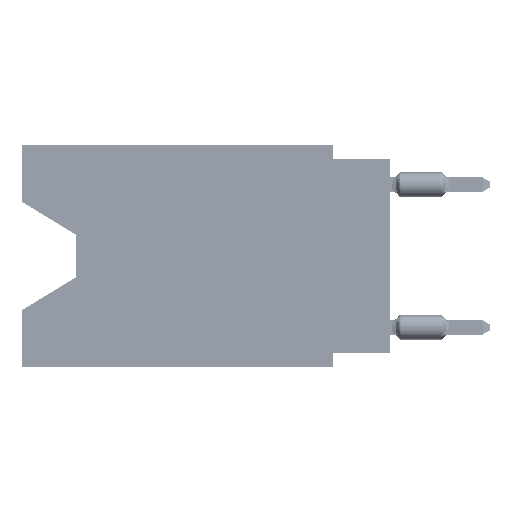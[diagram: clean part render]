
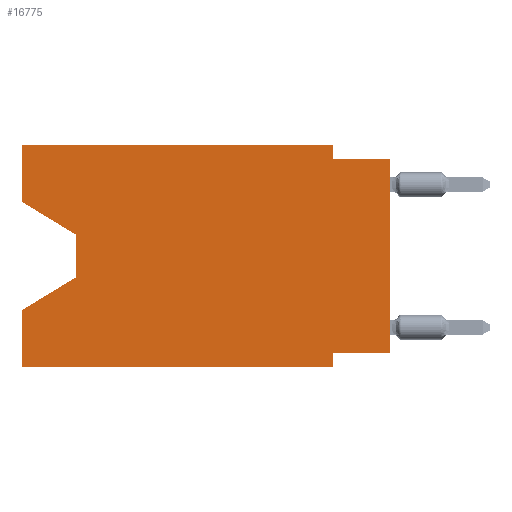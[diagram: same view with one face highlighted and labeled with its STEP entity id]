
A CAD part, left-side view. The second image highlights one B-rep face of the part: STEP entity #16775.
In plain terms, the highlighted planar face has unit normal (-1, 0, 0).
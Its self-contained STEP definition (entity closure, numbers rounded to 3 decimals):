
#1108 = CARTESIAN_POINT ( 'NONE',  ( 0., 16.383, -7.36 ) ) ;
#1515 = VECTOR ( 'NONE', #27946, 1000. ) ;
#1845 = EDGE_CURVE ( 'NONE', #78045, #65738, #79891, .T. ) ;
#3130 = CARTESIAN_POINT ( 'NONE',  ( 0., 16.383, 0. ) ) ;
#3333 = EDGE_CURVE ( 'NONE', #61982, #33048, #48291, .T. ) ;
#3709 = CARTESIAN_POINT ( 'NONE',  ( 0., 2.54, 0. ) ) ;
#4247 = LINE ( 'NONE', #18133, #17586 ) ;
#6754 = EDGE_CURVE ( 'NONE', #19609, #62767, #4247, .T. ) ;
#7972 = LINE ( 'NONE', #22274, #1515 ) ;
#8354 = DIRECTION ( 'NONE',  ( 0., 0., -1. ) ) ;
#8717 = LINE ( 'NONE', #36454, #43892 ) ;
#9831 = VECTOR ( 'NONE', #17596, 1000. ) ;
#12646 = CARTESIAN_POINT ( 'NONE',  ( 0., 16.383, 0. ) ) ;
#13495 = CARTESIAN_POINT ( 'NONE',  ( 0., 0., -0.635 ) ) ;
#13718 = CARTESIAN_POINT ( 'NONE',  ( 0., 13.97, -5.893 ) ) ;
#15014 = DIRECTION ( 'NONE',  ( 0., -1., 0. ) ) ;
#16775 = ADVANCED_FACE ( 'NONE', ( #78257 ), #64792, .F. ) ;
#17586 = VECTOR ( 'NONE', #44601, 1000. ) ;
#17596 = DIRECTION ( 'NONE',  ( 0., 0., -1. ) ) ;
#18133 = CARTESIAN_POINT ( 'NONE',  ( 0., 13.97, -4.013 ) ) ;
#18489 = VECTOR ( 'NONE', #82937, 1000. ) ;
#18749 = DIRECTION ( 'NONE',  ( 0., 0., -1. ) ) ;
#18790 = ORIENTED_EDGE ( 'NONE', *, *, #85277, .T. ) ;
#19493 = ORIENTED_EDGE ( 'NONE', *, *, #3333, .F. ) ;
#19609 = VERTEX_POINT ( 'NONE', #43507 ) ;
#20093 = CARTESIAN_POINT ( 'NONE',  ( 0., 2.54, -9.906 ) ) ;
#20587 = VECTOR ( 'NONE', #29185, 1000. ) ;
#20881 = ORIENTED_EDGE ( 'NONE', *, *, #49414, .F. ) ;
#21984 = EDGE_CURVE ( 'NONE', #61050, #45121, #60635, .T. ) ;
#22274 = CARTESIAN_POINT ( 'NONE',  ( 0., 0., -9.271 ) ) ;
#24250 = CARTESIAN_POINT ( 'NONE',  ( 0., 2.54, -9.271 ) ) ;
#24397 = LINE ( 'NONE', #49589, #58509 ) ;
#25466 = LINE ( 'NONE', #13718, #51421 ) ;
#25630 = ORIENTED_EDGE ( 'NONE', *, *, #6754, .T. ) ;
#26469 = CARTESIAN_POINT ( 'NONE',  ( 0., 2.54, 0. ) ) ;
#27946 = DIRECTION ( 'NONE',  ( 0., 1., 0. ) ) ;
#28156 = DIRECTION ( 'NONE',  ( 0., 0., 1. ) ) ;
#29185 = DIRECTION ( 'NONE',  ( 0., -1., 0. ) ) ;
#30332 = LINE ( 'NONE', #49467, #18489 ) ;
#33048 = VERTEX_POINT ( 'NONE', #20093 ) ;
#33711 = CARTESIAN_POINT ( 'NONE',  ( 0., 16.383, 0. ) ) ;
#33795 = CARTESIAN_POINT ( 'NONE',  ( 0., 16.383, 0. ) ) ;
#36454 = CARTESIAN_POINT ( 'NONE',  ( 0., 0., 0. ) ) ;
#36660 = LINE ( 'NONE', #48002, #85821 ) ;
#36768 = ORIENTED_EDGE ( 'NONE', *, *, #56775, .T. ) ;
#37767 = VERTEX_POINT ( 'NONE', #26469 ) ;
#38021 = VECTOR ( 'NONE', #28156, 1000. ) ;
#41029 = ORIENTED_EDGE ( 'NONE', *, *, #65079, .T. ) ;
#41229 = ORIENTED_EDGE ( 'NONE', *, *, #1845, .F. ) ;
#43507 = CARTESIAN_POINT ( 'NONE',  ( 0., 13.97, -4.013 ) ) ;
#43892 = VECTOR ( 'NONE', #61683, 1000. ) ;
#43999 = CARTESIAN_POINT ( 'NONE',  ( 0., 16.383, -9.906 ) ) ;
#44601 = DIRECTION ( 'NONE',  ( 0., 0., -1. ) ) ;
#45121 = VERTEX_POINT ( 'NONE', #1108 ) ;
#46500 = EDGE_CURVE ( 'NONE', #37767, #75358, #50590, .T. ) ;
#46737 = EDGE_CURVE ( 'NONE', #79454, #61982, #7972, .T. ) ;
#46905 = EDGE_CURVE ( 'NONE', #62767, #45121, #25466, .T. ) ;
#47860 = CARTESIAN_POINT ( 'NONE',  ( 0., 2.54, -9.906 ) ) ;
#48002 = CARTESIAN_POINT ( 'NONE',  ( 0., 16.383, -9.906 ) ) ;
#48291 = LINE ( 'NONE', #47860, #64580 ) ;
#48818 = CARTESIAN_POINT ( 'NONE',  ( 0., 0., -9.271 ) ) ;
#49414 = EDGE_CURVE ( 'NONE', #75358, #72971, #30332, .T. ) ;
#49467 = CARTESIAN_POINT ( 'NONE',  ( 0., 0., -0.635 ) ) ;
#49589 = CARTESIAN_POINT ( 'NONE',  ( 0., 16.383, -2.546 ) ) ;
#50590 = LINE ( 'NONE', #3709, #9831 ) ;
#50895 = DIRECTION ( 'NONE',  ( 0., -0.855, -0.519 ) ) ;
#51421 = VECTOR ( 'NONE', #79323, 1000. ) ;
#52121 = ORIENTED_EDGE ( 'NONE', *, *, #46737, .F. ) ;
#56775 = EDGE_CURVE ( 'NONE', #79454, #72971, #8717, .T. ) ;
#56961 = ORIENTED_EDGE ( 'NONE', *, *, #46500, .F. ) ;
#58368 = ORIENTED_EDGE ( 'NONE', *, *, #21984, .F. ) ;
#58509 = VECTOR ( 'NONE', #50895, 1000. ) ;
#59257 = EDGE_CURVE ( 'NONE', #65738, #37767, #69573, .T. ) ;
#59350 = DIRECTION ( 'NONE',  ( 0., 0., 1. ) ) ;
#59527 = AXIS2_PLACEMENT_3D ( 'NONE', #12646, #64355, #18749 ) ;
#60635 = LINE ( 'NONE', #33711, #68288 ) ;
#61050 = VERTEX_POINT ( 'NONE', #43999 ) ;
#61683 = DIRECTION ( 'NONE',  ( 0., 0., 1. ) ) ;
#61982 = VERTEX_POINT ( 'NONE', #24250 ) ;
#62767 = VERTEX_POINT ( 'NONE', #69658 ) ;
#64355 = DIRECTION ( 'NONE',  ( 1., 0., 0. ) ) ;
#64580 = VECTOR ( 'NONE', #8354, 1000. ) ;
#64792 = PLANE ( 'NONE',  #59527 ) ;
#65079 = EDGE_CURVE ( 'NONE', #78045, #19609, #24397, .T. ) ;
#65738 = VERTEX_POINT ( 'NONE', #81151 ) ;
#68288 = VECTOR ( 'NONE', #59350, 1000. ) ;
#69573 = LINE ( 'NONE', #3130, #20587 ) ;
#69658 = CARTESIAN_POINT ( 'NONE',  ( 0., 13.97, -5.893 ) ) ;
#72269 = CARTESIAN_POINT ( 'NONE',  ( 0., 2.54, -0.635 ) ) ;
#72629 = ORIENTED_EDGE ( 'NONE', *, *, #46905, .T. ) ;
#72971 = VERTEX_POINT ( 'NONE', #13495 ) ;
#75358 = VERTEX_POINT ( 'NONE', #72269 ) ;
#77151 = CARTESIAN_POINT ( 'NONE',  ( 0., 16.383, -2.546 ) ) ;
#78045 = VERTEX_POINT ( 'NONE', #77151 ) ;
#78257 = FACE_OUTER_BOUND ( 'NONE', #78830, .T. ) ;
#78830 = EDGE_LOOP ( 'NONE', ( #41029, #25630, #72629, #58368, #18790, #19493, #52121, #36768, #20881, #56961, #83514, #41229 ) ) ;
#79323 = DIRECTION ( 'NONE',  ( 0., 0.855, -0.519 ) ) ;
#79454 = VERTEX_POINT ( 'NONE', #48818 ) ;
#79891 = LINE ( 'NONE', #33795, #38021 ) ;
#81151 = CARTESIAN_POINT ( 'NONE',  ( 0., 16.383, 0. ) ) ;
#82937 = DIRECTION ( 'NONE',  ( 0., -1., 0. ) ) ;
#83514 = ORIENTED_EDGE ( 'NONE', *, *, #59257, .F. ) ;
#85277 = EDGE_CURVE ( 'NONE', #61050, #33048, #36660, .T. ) ;
#85821 = VECTOR ( 'NONE', #15014, 1000. ) ;
